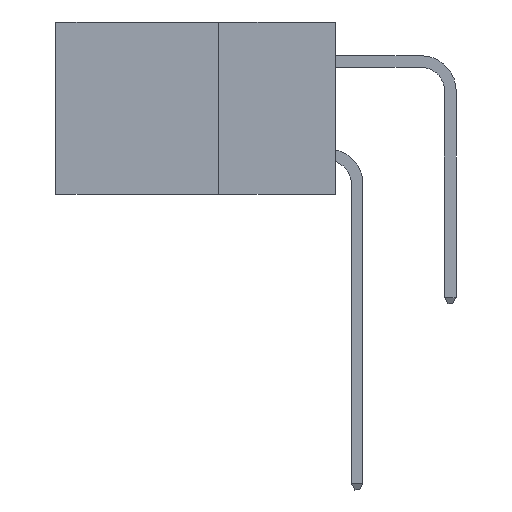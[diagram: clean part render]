
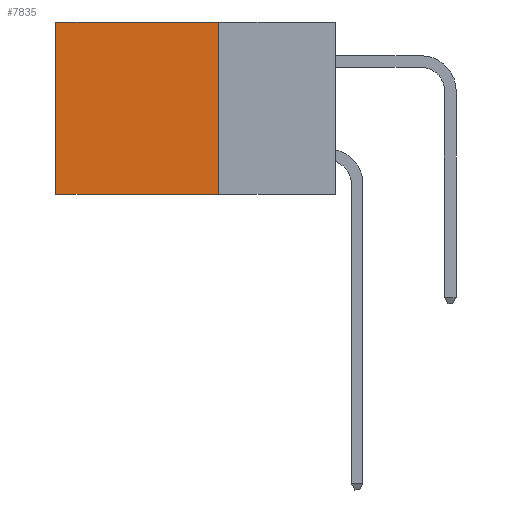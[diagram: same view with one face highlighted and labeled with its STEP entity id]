
A CAD part, left-side view. The second image highlights one B-rep face of the part: STEP entity #7835.
In plain terms, the highlighted planar face has unit normal (-1, 0, 0).
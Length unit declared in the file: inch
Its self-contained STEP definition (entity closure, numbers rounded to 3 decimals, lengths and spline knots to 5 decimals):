
#994 = CARTESIAN_POINT ( 'NONE',  ( 0.2875, 0.25, -0.37 ) ) ;
#1921 = FACE_OUTER_BOUND ( 'NONE', #7977, .T. ) ;
#4539 = VERTEX_POINT ( 'NONE', #994 ) ;
#5654 = DIRECTION ( 'NONE',  ( 0., 1., 0. ) ) ;
#5760 = DIRECTION ( 'NONE',  ( 0., 0., -1. ) ) ;
#6084 = LINE ( 'NONE', #19316, #23192 ) ;
#6636 = DIRECTION ( 'NONE',  ( 0., 0., -1. ) ) ;
#7835 = ADVANCED_FACE ( 'NONE', ( #1921 ), #9833, .F. ) ;
#7977 = EDGE_LOOP ( 'NONE', ( #11596, #13225, #19814, #8615 ) ) ;
#8020 = CARTESIAN_POINT ( 'NONE',  ( 0.2875, 0.25, 0. ) ) ;
#8144 = EDGE_CURVE ( 'NONE', #26247, #30388, #29967, .T. ) ;
#8268 = LINE ( 'NONE', #17047, #21563 ) ;
#8615 = ORIENTED_EDGE ( 'NONE', *, *, #8144, .T. ) ;
#9738 = VERTEX_POINT ( 'NONE', #17522 ) ;
#9833 = PLANE ( 'NONE',  #10792 ) ;
#10792 = AXIS2_PLACEMENT_3D ( 'NONE', #19423, #19200, #26541 ) ;
#11596 = ORIENTED_EDGE ( 'NONE', *, *, #19558, .T. ) ;
#13225 = ORIENTED_EDGE ( 'NONE', *, *, #15142, .F. ) ;
#14812 = VECTOR ( 'NONE', #5654, 39.37008 ) ;
#15142 = EDGE_CURVE ( 'NONE', #4539, #9738, #8268, .T. ) ;
#17047 = CARTESIAN_POINT ( 'NONE',  ( 0.2875, 0.25, -0.37 ) ) ;
#17522 = CARTESIAN_POINT ( 'NONE',  ( 0.2875, 0.6, -0.37 ) ) ;
#19200 = DIRECTION ( 'NONE',  ( 1., 0., 0. ) ) ;
#19313 = CARTESIAN_POINT ( 'NONE',  ( 0.2875, 0.6, 0. ) ) ;
#19316 = CARTESIAN_POINT ( 'NONE',  ( 0.2875, 0.6, 0. ) ) ;
#19419 = LINE ( 'NONE', #28310, #25062 ) ;
#19423 = CARTESIAN_POINT ( 'NONE',  ( 0.2875, 0.25, 0. ) ) ;
#19558 = EDGE_CURVE ( 'NONE', #30388, #9738, #6084, .T. ) ;
#19814 = ORIENTED_EDGE ( 'NONE', *, *, #29142, .F. ) ;
#21563 = VECTOR ( 'NONE', #24882, 39.37008 ) ;
#21783 = CARTESIAN_POINT ( 'NONE',  ( 0.2875, 0.25, 0. ) ) ;
#23192 = VECTOR ( 'NONE', #5760, 39.37008 ) ;
#24882 = DIRECTION ( 'NONE',  ( 0., 1., 0. ) ) ;
#25062 = VECTOR ( 'NONE', #6636, 39.37008 ) ;
#26247 = VERTEX_POINT ( 'NONE', #21783 ) ;
#26541 = DIRECTION ( 'NONE',  ( 0., 0., -1. ) ) ;
#28310 = CARTESIAN_POINT ( 'NONE',  ( 0.2875, 0.25, 0. ) ) ;
#29142 = EDGE_CURVE ( 'NONE', #26247, #4539, #19419, .T. ) ;
#29967 = LINE ( 'NONE', #8020, #14812 ) ;
#30388 = VERTEX_POINT ( 'NONE', #19313 ) ;
